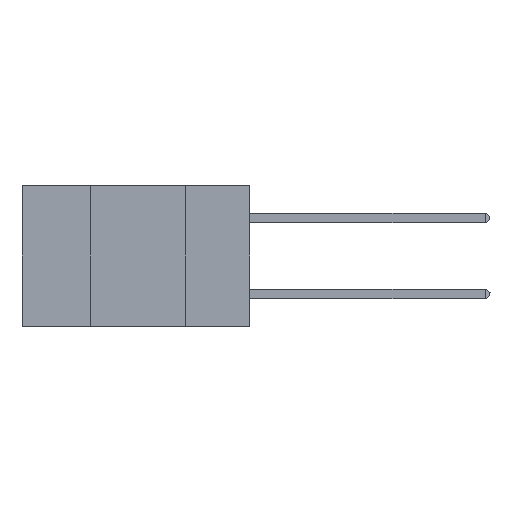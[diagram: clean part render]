
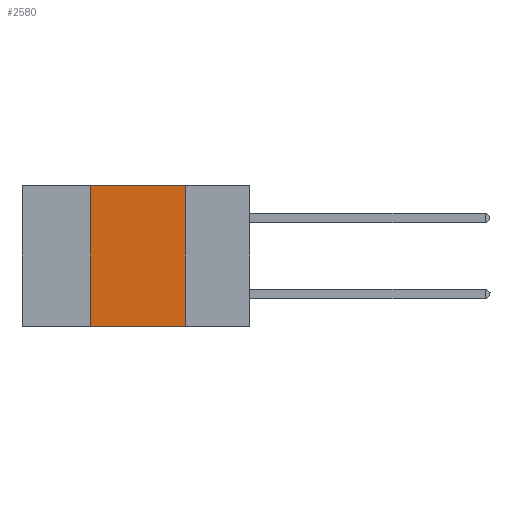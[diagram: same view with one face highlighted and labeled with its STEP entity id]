
A CAD part, left-side view. The second image highlights one B-rep face of the part: STEP entity #2580.
In plain terms, the highlighted planar face has unit normal (-1, 0, 0).
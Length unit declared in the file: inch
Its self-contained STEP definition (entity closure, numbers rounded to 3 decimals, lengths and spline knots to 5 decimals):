
#1224 = VERTEX_POINT ( 'NONE', #20726 ) ;
#2320 = VECTOR ( 'NONE', #25928, 39.37008 ) ;
#2580 = ADVANCED_FACE ( 'NONE', ( #13008 ), #11068, .F. ) ;
#3598 = LINE ( 'NONE', #16105, #19012 ) ;
#4424 = LINE ( 'NONE', #13057, #14494 ) ;
#5005 = DIRECTION ( 'NONE',  ( 0., 0., -1. ) ) ;
#5258 = LINE ( 'NONE', #12624, #25873 ) ;
#6108 = DIRECTION ( 'NONE',  ( 0., -1., 0. ) ) ;
#7029 = CARTESIAN_POINT ( 'NONE',  ( 0., 0.6, 0. ) ) ;
#10924 = ORIENTED_EDGE ( 'NONE', *, *, #16582, .T. ) ;
#11068 = PLANE ( 'NONE',  #13202 ) ;
#11177 = ORIENTED_EDGE ( 'NONE', *, *, #11546, .F. ) ;
#11546 = EDGE_CURVE ( 'NONE', #16637, #13844, #5258, .T. ) ;
#11589 = VERTEX_POINT ( 'NONE', #14765 ) ;
#12624 = CARTESIAN_POINT ( 'NONE',  ( 0., 0.17, 0. ) ) ;
#13008 = FACE_OUTER_BOUND ( 'NONE', #16763, .T. ) ;
#13057 = CARTESIAN_POINT ( 'NONE',  ( 0., 0.42, 0. ) ) ;
#13202 = AXIS2_PLACEMENT_3D ( 'NONE', #7029, #19041, #5005 ) ;
#13844 = VERTEX_POINT ( 'NONE', #17519 ) ;
#14494 = VECTOR ( 'NONE', #15044, 39.37008 ) ;
#14765 = CARTESIAN_POINT ( 'NONE',  ( 0., 0.42, -0.37 ) ) ;
#15044 = DIRECTION ( 'NONE',  ( 0., 0., 1. ) ) ;
#16105 = CARTESIAN_POINT ( 'NONE',  ( 0., 0.6, -0.37 ) ) ;
#16582 = EDGE_CURVE ( 'NONE', #11589, #13844, #3598, .T. ) ;
#16637 = VERTEX_POINT ( 'NONE', #24297 ) ;
#16763 = EDGE_LOOP ( 'NONE', ( #11177, #24650, #20677, #10924 ) ) ;
#17519 = CARTESIAN_POINT ( 'NONE',  ( 0., 0.17, -0.37 ) ) ;
#18393 = LINE ( 'NONE', #23954, #2320 ) ;
#19012 = VECTOR ( 'NONE', #6108, 39.37008 ) ;
#19041 = DIRECTION ( 'NONE',  ( 1., 0., 0. ) ) ;
#20587 = EDGE_CURVE ( 'NONE', #11589, #1224, #4424, .T. ) ;
#20677 = ORIENTED_EDGE ( 'NONE', *, *, #20587, .F. ) ;
#20726 = CARTESIAN_POINT ( 'NONE',  ( 0., 0.42, 0. ) ) ;
#22632 = DIRECTION ( 'NONE',  ( 0., 0., -1. ) ) ;
#23954 = CARTESIAN_POINT ( 'NONE',  ( 0., 0.6, 0. ) ) ;
#24210 = EDGE_CURVE ( 'NONE', #1224, #16637, #18393, .T. ) ;
#24297 = CARTESIAN_POINT ( 'NONE',  ( 0., 0.17, 0. ) ) ;
#24650 = ORIENTED_EDGE ( 'NONE', *, *, #24210, .F. ) ;
#25873 = VECTOR ( 'NONE', #22632, 39.37008 ) ;
#25928 = DIRECTION ( 'NONE',  ( 0., -1., 0. ) ) ;
